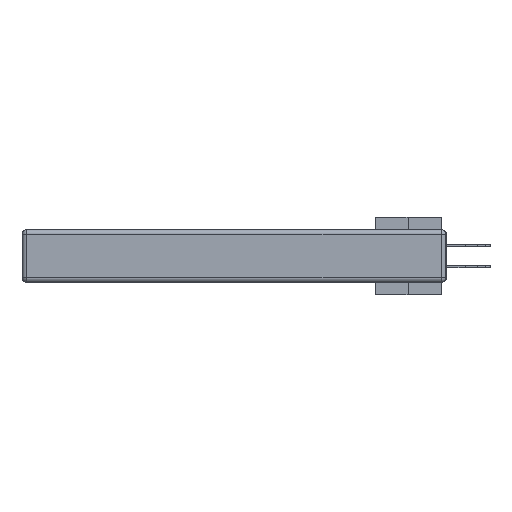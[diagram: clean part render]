
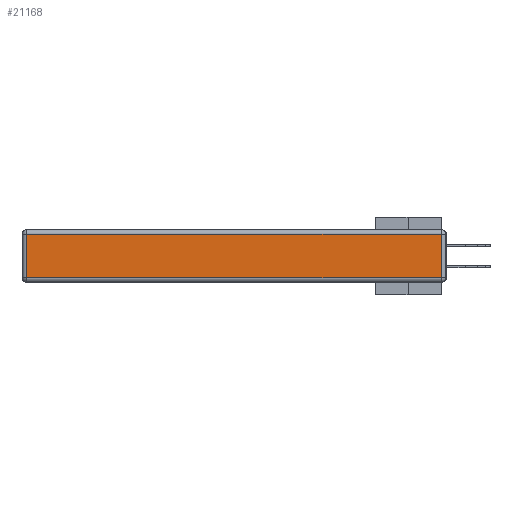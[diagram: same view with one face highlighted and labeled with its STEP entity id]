
A CAD part, left-side view. The second image highlights one B-rep face of the part: STEP entity #21168.
In plain terms, the highlighted planar face has unit normal (-1, 0, 0).
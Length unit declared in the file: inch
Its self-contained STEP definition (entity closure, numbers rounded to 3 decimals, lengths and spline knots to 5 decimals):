
#434 = FACE_OUTER_BOUND ( 'NONE', #13179, .T. ) ;
#626 = VERTEX_POINT ( 'NONE', #27137 ) ;
#652 = ORIENTED_EDGE ( 'NONE', *, *, #21381, .T. ) ;
#878 = VERTEX_POINT ( 'NONE', #26594 ) ;
#1499 = CARTESIAN_POINT ( 'NONE',  ( 0., 2.72, -0.343 ) ) ;
#5963 = EDGE_CURVE ( 'NONE', #12274, #878, #23026, .T. ) ;
#6551 = PLANE ( 'NONE',  #36685 ) ;
#6629 = VECTOR ( 'NONE', #36831, 39.37008 ) ;
#7347 = VECTOR ( 'NONE', #18991, 39.37008 ) ;
#9670 = DIRECTION ( 'NONE',  ( -1., 0., 0. ) ) ;
#10674 = VECTOR ( 'NONE', #38465, 39.37008 ) ;
#11169 = VERTEX_POINT ( 'NONE', #27969 ) ;
#12011 = ORIENTED_EDGE ( 'NONE', *, *, #5963, .T. ) ;
#12274 = VERTEX_POINT ( 'NONE', #25024 ) ;
#13179 = EDGE_LOOP ( 'NONE', ( #652, #30430, #12011, #35120 ) ) ;
#14219 = VECTOR ( 'NONE', #17702, 39.37008 ) ;
#16379 = EDGE_CURVE ( 'NONE', #11169, #12274, #38128, .T. ) ;
#17702 = DIRECTION ( 'NONE',  ( 0., 1., 0. ) ) ;
#18991 = DIRECTION ( 'NONE',  ( 0., 0., 1. ) ) ;
#19990 = LINE ( 'NONE', #31458, #10674 ) ;
#20819 = CARTESIAN_POINT ( 'NONE',  ( 0., 2.75, -0.03 ) ) ;
#21168 = ADVANCED_FACE ( 'NONE', ( #434 ), #6551, .T. ) ;
#21381 = EDGE_CURVE ( 'NONE', #626, #11169, #19990, .T. ) ;
#23026 = LINE ( 'NONE', #20819, #14219 ) ;
#25024 = CARTESIAN_POINT ( 'NONE',  ( 0., 0.03, -0.03 ) ) ;
#26211 = LINE ( 'NONE', #1499, #6629 ) ;
#26594 = CARTESIAN_POINT ( 'NONE',  ( 0., 2.72, -0.03 ) ) ;
#27137 = CARTESIAN_POINT ( 'NONE',  ( 0., 2.72, -0.313 ) ) ;
#27969 = CARTESIAN_POINT ( 'NONE',  ( 0., 0.03, -0.313 ) ) ;
#29397 = EDGE_CURVE ( 'NONE', #878, #626, #26211, .T. ) ;
#30430 = ORIENTED_EDGE ( 'NONE', *, *, #16379, .T. ) ;
#30806 = CARTESIAN_POINT ( 'NONE',  ( 0., 0.03, -0.343 ) ) ;
#31458 = CARTESIAN_POINT ( 'NONE',  ( 0., 0., -0.313 ) ) ;
#33604 = DIRECTION ( 'NONE',  ( 0., 0., 1. ) ) ;
#35120 = ORIENTED_EDGE ( 'NONE', *, *, #29397, .T. ) ;
#36366 = CARTESIAN_POINT ( 'NONE',  ( 0., 0., -0.343 ) ) ;
#36685 = AXIS2_PLACEMENT_3D ( 'NONE', #36366, #9670, #33604 ) ;
#36831 = DIRECTION ( 'NONE',  ( 0., 0., -1. ) ) ;
#38128 = LINE ( 'NONE', #30806, #7347 ) ;
#38465 = DIRECTION ( 'NONE',  ( 0., -1., 0. ) ) ;
